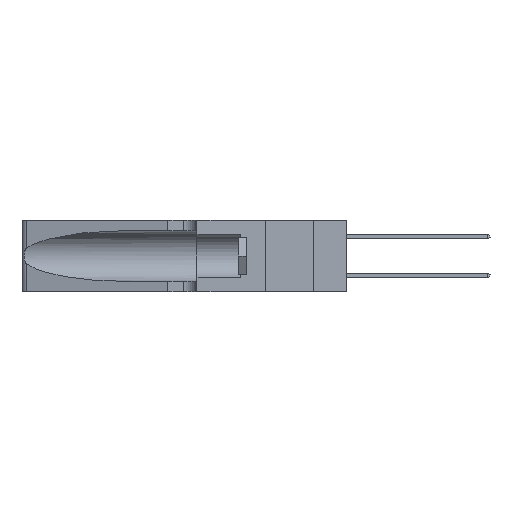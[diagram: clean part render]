
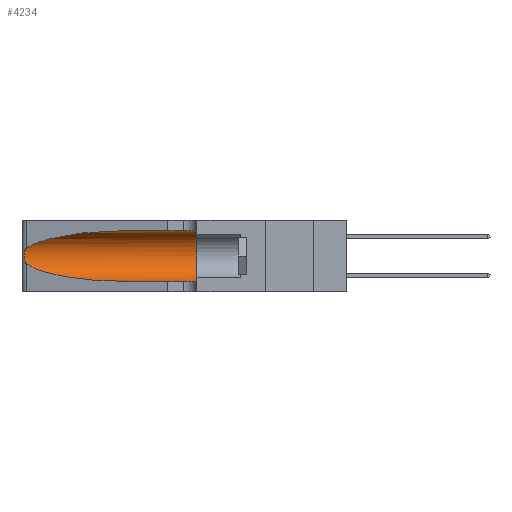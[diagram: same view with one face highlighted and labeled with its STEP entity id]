
A CAD part, left-side view. The second image highlights one B-rep face of the part: STEP entity #4234.
In plain terms, the highlighted cylindrical face has radius 3.308 mm (diameter 6.617 mm), a partial arc.
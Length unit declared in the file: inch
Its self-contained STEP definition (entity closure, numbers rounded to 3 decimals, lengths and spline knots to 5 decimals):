
#700 = CARTESIAN_POINT ( 'NONE',  ( 0.1305, 0.72297, 0.05475 ) ) ;
#1132 = CARTESIAN_POINT ( 'NONE',  ( 0.25487, 1.22718, 0.22369 ) ) ;
#1186 = DIRECTION ( 'NONE',  ( 0., 0., -1. ) ) ;
#1491 = DIRECTION ( 'NONE',  ( 0., 1., 0. ) ) ;
#1734 = DIRECTION ( 'NONE',  ( 0., -1., 0. ) ) ;
#1748 = CARTESIAN_POINT ( 'NONE',  ( 0.25639, 1.23184, 0.21858 ) ) ;
#2003 = VECTOR ( 'NONE', #3818, 39.37008 ) ;
#2251 = EDGE_CURVE ( 'NONE', #14916, #18921, #22269, .T. ) ;
#3282 = ORIENTED_EDGE ( 'NONE', *, *, #14587, .T. ) ;
#3708 = CARTESIAN_POINT ( 'NONE',  ( 0.25854, 1.2359, 0.20912 ) ) ;
#3736 = CARTESIAN_POINT ( 'NONE',  ( 0.1305, 0.35, 0.05475 ) ) ;
#3818 = DIRECTION ( 'NONE',  ( 0., -1., 0. ) ) ;
#4234 = ADVANCED_FACE ( 'NONE', ( #13811 ), #17818, .F. ) ;
#4556 = CARTESIAN_POINT ( 'NONE',  ( 0.25487, 1.22718, 0.14631 ) ) ;
#4850 =( BOUNDED_CURVE ( )  B_SPLINE_CURVE ( 3, ( #4556, #22235, #12461, #700 ),
 .UNSPECIFIED., .F., .T. ) 
 B_SPLINE_CURVE_WITH_KNOTS ( ( 4, 4 ),
 ( 3.44316, 4.71239 ),
 .UNSPECIFIED. ) 
 CURVE ( )  GEOMETRIC_REPRESENTATION_ITEM ( )  RATIONAL_B_SPLINE_CURVE ( ( 1., 0.87, 0.87, 1. ) ) 
 REPRESENTATION_ITEM ( '' )  );
#5202 = CARTESIAN_POINT ( 'NONE',  ( 0.18966, 0.96281, 0.31525 ) ) ;
#5411 = VERTEX_POINT ( 'NONE', #1132 ) ;
#5498 = CARTESIAN_POINT ( 'NONE',  ( 0.1305, 0.35, 0.31525 ) ) ;
#5568 = EDGE_CURVE ( 'NONE', #5411, #23649, #23190, .T. ) ;
#5680 = CARTESIAN_POINT ( 'NONE',  ( 0.26075, 1.23896, 0.19203 ) ) ;
#5826 = VERTEX_POINT ( 'NONE', #24195 ) ;
#5928 = VECTOR ( 'NONE', #1734, 39.37008 ) ;
#6701 = EDGE_CURVE ( 'NONE', #5826, #5411, #13989, .T. ) ;
#7229 = CARTESIAN_POINT ( 'NONE',  ( 0.2373, 1.15595, 0.28018 ) ) ;
#7625 = CARTESIAN_POINT ( 'NONE',  ( 0.25487, 1.22718, 0.14631 ) ) ;
#7637 = CARTESIAN_POINT ( 'NONE',  ( 0.26017, 1.23833, 0.17102 ) ) ;
#7680 = VERTEX_POINT ( 'NONE', #11590 ) ;
#9609 = CARTESIAN_POINT ( 'NONE',  ( 0.25789, 1.23486, 0.15765 ) ) ;
#11136 = LINE ( 'NONE', #25316, #5928 ) ;
#11506 = CARTESIAN_POINT ( 'NONE',  ( 0.25487, 1.22718, 0.22369 ) ) ;
#11590 = CARTESIAN_POINT ( 'NONE',  ( 0.1305, 0.72297, 0.05475 ) ) ;
#11600 = CARTESIAN_POINT ( 'NONE',  ( 0.25555, 1.22993, 0.14849 ) ) ;
#12143 = EDGE_CURVE ( 'NONE', #7680, #18921, #11136, .T. ) ;
#12461 = CARTESIAN_POINT ( 'NONE',  ( 0.18966, 0.96281, 0.05475 ) ) ;
#13249 = CARTESIAN_POINT ( 'NONE',  ( 0.1305, 0.35, 0.185 ) ) ;
#13456 = ORIENTED_EDGE ( 'NONE', *, *, #18942, .F. ) ;
#13504 = CARTESIAN_POINT ( 'NONE',  ( 0.25555, 1.22994, 0.2215 ) ) ;
#13612 = CARTESIAN_POINT ( 'NONE',  ( 0.1305, 1.61858, 0.31525 ) ) ;
#13811 = FACE_OUTER_BOUND ( 'NONE', #22419, .T. ) ;
#13989 =( BOUNDED_CURVE ( )  B_SPLINE_CURVE ( 3, ( #20969, #5202, #7229, #21060 ),
 .UNSPECIFIED., .F., .F. ) 
 B_SPLINE_CURVE_WITH_KNOTS ( ( 4, 4 ),
 ( 1.5708, 2.84003 ),
 .UNSPECIFIED. ) 
 CURVE ( )  GEOMETRIC_REPRESENTATION_ITEM ( )  RATIONAL_B_SPLINE_CURVE ( ( 1., 0.87, 0.87, 1. ) ) 
 REPRESENTATION_ITEM ( '' )  );
#14587 = EDGE_CURVE ( 'NONE', #23649, #7680, #4850, .T. ) ;
#14916 = VERTEX_POINT ( 'NONE', #5498 ) ;
#14919 = DIRECTION ( 'NONE',  ( 0., -1., 0. ) ) ;
#15217 = DIRECTION ( 'NONE',  ( 0., 0., 1. ) ) ;
#15463 = CARTESIAN_POINT ( 'NONE',  ( 0.25787, 1.23484, 0.2124 ) ) ;
#15886 = ORIENTED_EDGE ( 'NONE', *, *, #6701, .T. ) ;
#16507 = ORIENTED_EDGE ( 'NONE', *, *, #5568, .T. ) ;
#16909 = CARTESIAN_POINT ( 'NONE',  ( 0.1305, 1.61858, 0.185 ) ) ;
#17462 = CARTESIAN_POINT ( 'NONE',  ( 0.26018, 1.23835, 0.19895 ) ) ;
#17682 = LINE ( 'NONE', #13612, #2003 ) ;
#17818 = CYLINDRICAL_SURFACE ( 'NONE', #24798, 0.13025 ) ;
#18087 = ORIENTED_EDGE ( 'NONE', *, *, #2251, .F. ) ;
#18477 = AXIS2_PLACEMENT_3D ( 'NONE', #13249, #1491, #15217 ) ;
#18921 = VERTEX_POINT ( 'NONE', #3736 ) ;
#18942 = EDGE_CURVE ( 'NONE', #5826, #14916, #17682, .T. ) ;
#19480 = CARTESIAN_POINT ( 'NONE',  ( 0.26075, 1.23896, 0.178 ) ) ;
#20261 = ORIENTED_EDGE ( 'NONE', *, *, #12143, .T. ) ;
#20969 = CARTESIAN_POINT ( 'NONE',  ( 0.1305, 0.72297, 0.31525 ) ) ;
#21060 = CARTESIAN_POINT ( 'NONE',  ( 0.25487, 1.22718, 0.22369 ) ) ;
#21478 = CARTESIAN_POINT ( 'NONE',  ( 0.25856, 1.23593, 0.16098 ) ) ;
#22235 = CARTESIAN_POINT ( 'NONE',  ( 0.2373, 1.15595, 0.08982 ) ) ;
#22269 = CIRCLE ( 'NONE', #18477, 0.13025 ) ;
#22419 = EDGE_LOOP ( 'NONE', ( #15886, #16507, #3282, #20261, #18087, #13456 ) ) ;
#23190 = B_SPLINE_CURVE_WITH_KNOTS ( 'NONE', 3,
 ( #11506, #13504, #1748, #15463, #3708, #17462, #5680, #19480, #7637, #21478, #9609, #23445, #11600, #25406 ),
 .UNSPECIFIED., .F., .F.,
 ( 4, 2, 2, 2, 2, 2, 4 ),
 ( 0., 0.00027, 0.00053, 0.00107, 0.0016, 0.00187, 0.00214 ),
 .UNSPECIFIED. ) ;
#23445 = CARTESIAN_POINT ( 'NONE',  ( 0.25639, 1.23186, 0.15144 ) ) ;
#23649 = VERTEX_POINT ( 'NONE', #7625 ) ;
#24195 = CARTESIAN_POINT ( 'NONE',  ( 0.1305, 0.72297, 0.31525 ) ) ;
#24798 = AXIS2_PLACEMENT_3D ( 'NONE', #16909, #14919, #1186 ) ;
#25316 = CARTESIAN_POINT ( 'NONE',  ( 0.1305, 1.61858, 0.05475 ) ) ;
#25406 = CARTESIAN_POINT ( 'NONE',  ( 0.25487, 1.22718, 0.14631 ) ) ;
